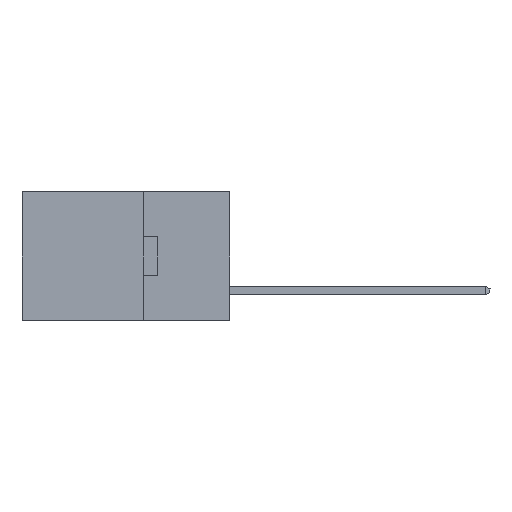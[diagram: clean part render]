
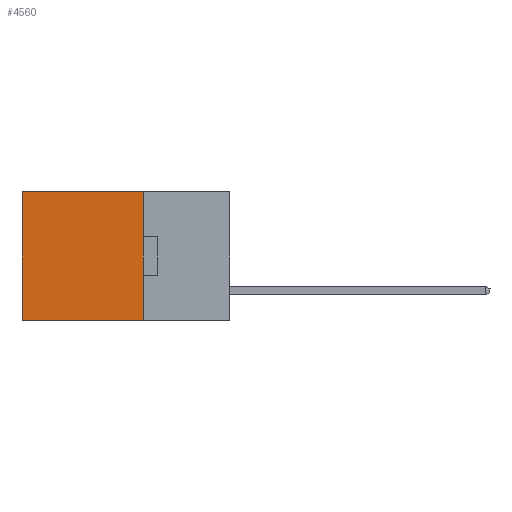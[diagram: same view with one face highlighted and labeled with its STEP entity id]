
A CAD part, left-side view. The second image highlights one B-rep face of the part: STEP entity #4560.
In plain terms, the highlighted planar face has unit normal (-1, 0, 0).
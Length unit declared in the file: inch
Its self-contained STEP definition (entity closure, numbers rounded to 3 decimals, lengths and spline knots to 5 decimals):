
#159 = ORIENTED_EDGE ( 'NONE', *, *, #16675, .T. ) ;
#512 = CARTESIAN_POINT ( 'NONE',  ( 0.2615, 0.6, -0.37 ) ) ;
#809 = CARTESIAN_POINT ( 'NONE',  ( 0.2615, 0.25, -0.37 ) ) ;
#1037 = ORIENTED_EDGE ( 'NONE', *, *, #4651, .F. ) ;
#1373 = VECTOR ( 'NONE', #13724, 39.37008 ) ;
#2558 = CARTESIAN_POINT ( 'NONE',  ( 0.2615, 0.25, 0. ) ) ;
#2842 = CARTESIAN_POINT ( 'NONE',  ( 0.2615, 0.25, 0. ) ) ;
#4190 = PLANE ( 'NONE',  #25237 ) ;
#4560 = ADVANCED_FACE ( 'NONE', ( #27096 ), #4190, .F. ) ;
#4651 = EDGE_CURVE ( 'NONE', #8258, #17584, #17355, .T. ) ;
#4812 = ORIENTED_EDGE ( 'NONE', *, *, #13789, .T. ) ;
#4901 = VECTOR ( 'NONE', #15021, 39.37008 ) ;
#5460 = LINE ( 'NONE', #809, #23257 ) ;
#6746 = DIRECTION ( 'NONE',  ( 0., 0., -1. ) ) ;
#6858 = EDGE_CURVE ( 'NONE', #22888, #8258, #5460, .T. ) ;
#8258 = VERTEX_POINT ( 'NONE', #9652 ) ;
#9652 = CARTESIAN_POINT ( 'NONE',  ( 0.2615, 0.25, -0.37 ) ) ;
#11156 = LINE ( 'NONE', #512, #4901 ) ;
#12368 = DIRECTION ( 'NONE',  ( 0., 0., -1. ) ) ;
#12497 = DIRECTION ( 'NONE',  ( 1., 0., 0. ) ) ;
#13724 = DIRECTION ( 'NONE',  ( 0., 1., 0. ) ) ;
#13789 = EDGE_CURVE ( 'NONE', #22888, #22382, #17526, .T. ) ;
#14065 = EDGE_LOOP ( 'NONE', ( #159, #1037, #22982, #4812 ) ) ;
#15021 = DIRECTION ( 'NONE',  ( 0., 0., -1. ) ) ;
#15856 = VECTOR ( 'NONE', #24300, 39.37008 ) ;
#16675 = EDGE_CURVE ( 'NONE', #22382, #17584, #11156, .T. ) ;
#17355 = LINE ( 'NONE', #21642, #1373 ) ;
#17526 = LINE ( 'NONE', #2842, #15856 ) ;
#17584 = VERTEX_POINT ( 'NONE', #20565 ) ;
#20565 = CARTESIAN_POINT ( 'NONE',  ( 0.2615, 0.6, -0.37 ) ) ;
#21191 = CARTESIAN_POINT ( 'NONE',  ( 0.2615, 0.6, 0. ) ) ;
#21642 = CARTESIAN_POINT ( 'NONE',  ( 0.2615, 0.25, -0.37 ) ) ;
#22382 = VERTEX_POINT ( 'NONE', #21191 ) ;
#22888 = VERTEX_POINT ( 'NONE', #2558 ) ;
#22982 = ORIENTED_EDGE ( 'NONE', *, *, #6858, .F. ) ;
#23257 = VECTOR ( 'NONE', #6746, 39.37008 ) ;
#24300 = DIRECTION ( 'NONE',  ( 0., 1., 0. ) ) ;
#25119 = CARTESIAN_POINT ( 'NONE',  ( 0.2615, 0.25, -0.37 ) ) ;
#25237 = AXIS2_PLACEMENT_3D ( 'NONE', #25119, #12497, #12368 ) ;
#27096 = FACE_OUTER_BOUND ( 'NONE', #14065, .T. ) ;
